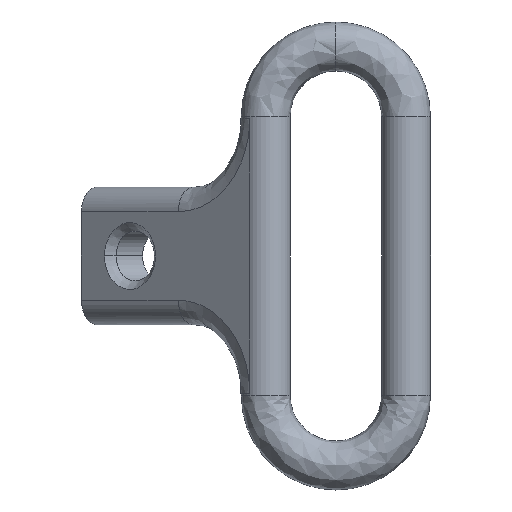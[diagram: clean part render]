
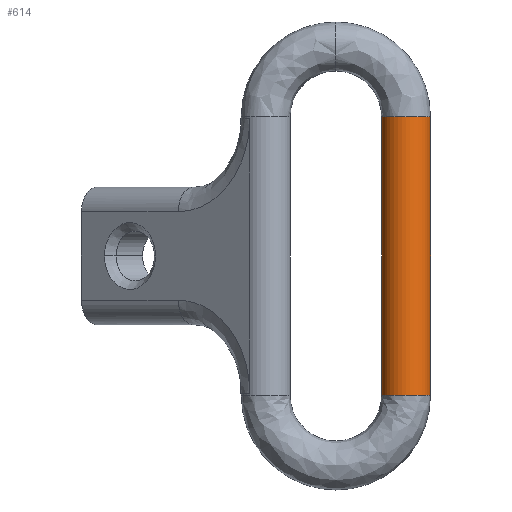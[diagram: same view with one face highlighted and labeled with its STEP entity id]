
A CAD part, front view. The second image highlights one B-rep face of the part: STEP entity #614.
In plain terms, the highlighted cylindrical face has radius 2.261 mm (diameter 4.521 mm), a partial arc.
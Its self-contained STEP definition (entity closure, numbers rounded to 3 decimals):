
#46 = DIRECTION ( 'NONE',  ( 0., 0., -1. ) ) ;
#95 = VERTEX_POINT ( 'NONE', #242 ) ;
#98 = VECTOR ( 'NONE', #46, 1000. ) ;
#178 = CIRCLE ( 'NONE', #458, 2.261 ) ;
#233 = CARTESIAN_POINT ( 'NONE',  ( 4.21, -0.025, 12.859 ) ) ;
#242 = CARTESIAN_POINT ( 'NONE',  ( 8.731, -0.025, -12.859 ) ) ;
#258 = ORIENTED_EDGE ( 'NONE', *, *, #911, .T. ) ;
#306 = FACE_OUTER_BOUND ( 'NONE', #676, .T. ) ;
#334 = LINE ( 'NONE', #842, #999 ) ;
#386 = VERTEX_POINT ( 'NONE', #233 ) ;
#428 = CARTESIAN_POINT ( 'NONE',  ( 6.471, -0.025, -12.859 ) ) ;
#458 = AXIS2_PLACEMENT_3D ( 'NONE', #428, #1336, #569 ) ;
#518 = ORIENTED_EDGE ( 'NONE', *, *, #1164, .T. ) ;
#553 = AXIS2_PLACEMENT_3D ( 'NONE', #883, #873, #865 ) ;
#569 = DIRECTION ( 'NONE',  ( -1., 0., 0. ) ) ;
#585 = AXIS2_PLACEMENT_3D ( 'NONE', #1165, #1106, #1110 ) ;
#614 = ADVANCED_FACE ( 'NONE', ( #306 ), #1491, .T. ) ;
#627 = ORIENTED_EDGE ( 'NONE', *, *, #1209, .F. ) ;
#676 = EDGE_LOOP ( 'NONE', ( #518, #1263, #258, #627 ) ) ;
#842 = CARTESIAN_POINT ( 'NONE',  ( 4.21, -0.025, 12.859 ) ) ;
#848 = CARTESIAN_POINT ( 'NONE',  ( 4.21, -0.025, -12.859 ) ) ;
#865 = DIRECTION ( 'NONE',  ( -1., 0., 0. ) ) ;
#873 = DIRECTION ( 'NONE',  ( 0., 0., -1. ) ) ;
#883 = CARTESIAN_POINT ( 'NONE',  ( 6.471, -0.025, 12.859 ) ) ;
#911 = EDGE_CURVE ( 'NONE', #1419, #386, #1045, .T. ) ;
#971 = DIRECTION ( 'NONE',  ( 0., 0., 1. ) ) ;
#999 = VECTOR ( 'NONE', #971, 1000. ) ;
#1035 = LINE ( 'NONE', #1473, #98 ) ;
#1045 = CIRCLE ( 'NONE', #553, 2.261 ) ;
#1106 = DIRECTION ( 'NONE',  ( 0., 0., -1. ) ) ;
#1110 = DIRECTION ( 'NONE',  ( -1., 0., 0. ) ) ;
#1164 = EDGE_CURVE ( 'NONE', #1437, #95, #178, .T. ) ;
#1165 = CARTESIAN_POINT ( 'NONE',  ( 6.471, -0.025, 12.859 ) ) ;
#1205 = EDGE_CURVE ( 'NONE', #1419, #95, #1035, .T. ) ;
#1209 = EDGE_CURVE ( 'NONE', #1437, #386, #334, .T. ) ;
#1263 = ORIENTED_EDGE ( 'NONE', *, *, #1205, .F. ) ;
#1336 = DIRECTION ( 'NONE',  ( 0., 0., 1. ) ) ;
#1419 = VERTEX_POINT ( 'NONE', #1482 ) ;
#1437 = VERTEX_POINT ( 'NONE', #848 ) ;
#1473 = CARTESIAN_POINT ( 'NONE',  ( 8.731, -0.025, 12.859 ) ) ;
#1482 = CARTESIAN_POINT ( 'NONE',  ( 8.731, -0.025, 12.859 ) ) ;
#1491 = CYLINDRICAL_SURFACE ( 'NONE', #585, 2.261 ) ;
